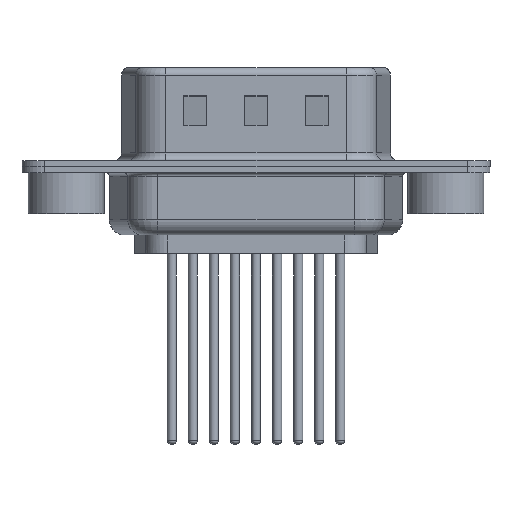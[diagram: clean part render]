
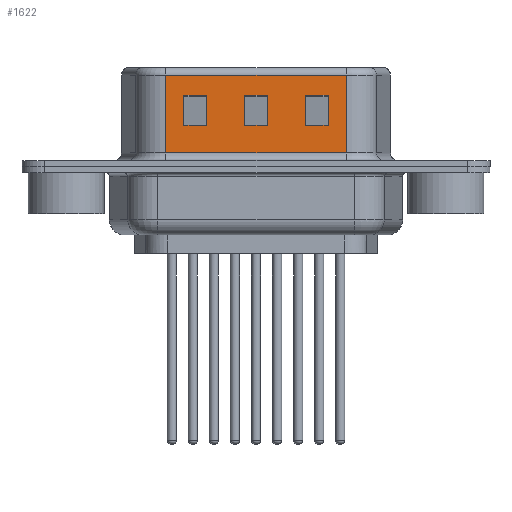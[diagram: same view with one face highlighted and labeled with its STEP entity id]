
A CAD part, front view. The second image highlights one B-rep face of the part: STEP entity #1622.
In plain terms, the highlighted planar face has unit normal (0, -1, 0).
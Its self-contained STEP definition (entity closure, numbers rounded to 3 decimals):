
#110 = CARTESIAN_POINT ( 'NONE',  ( 15.75, -4.55, 6.52 ) ) ;
#192 = CARTESIAN_POINT ( 'NONE',  ( 13.25, -4.55, 4.705 ) ) ;
#197 = EDGE_CURVE ( 'NONE', #6406, #1345, #12209, .T. ) ;
#223 = EDGE_CURVE ( 'NONE', #12306, #12247, #8976, .T. ) ;
#243 = CARTESIAN_POINT ( 'NONE',  ( 15.75, -4.55, 2.705 ) ) ;
#378 = DIRECTION ( 'NONE',  ( 1., 0., 0. ) ) ;
#596 = LINE ( 'NONE', #2812, #13760 ) ;
#843 = CARTESIAN_POINT ( 'NONE',  ( 13.25, -4.55, 6.52 ) ) ;
#916 = VERTEX_POINT ( 'NONE', #6265 ) ;
#1202 = FACE_OUTER_BOUND ( 'NONE', #9700, .T. ) ;
#1207 = EDGE_CURVE ( 'NONE', #12306, #9636, #13440, .T. ) ;
#1319 = LINE ( 'NONE', #5801, #10134 ) ;
#1322 = VECTOR ( 'NONE', #3563, 1000. ) ;
#1345 = VERTEX_POINT ( 'NONE', #10413 ) ;
#1435 = EDGE_CURVE ( 'NONE', #12232, #7040, #1764, .T. ) ;
#1436 = CARTESIAN_POINT ( 'NONE',  ( 7.75, -4.55, 6.52 ) ) ;
#1447 = VECTOR ( 'NONE', #6151, 1000. ) ;
#1486 = VECTOR ( 'NONE', #4485, 1000. ) ;
#1622 = ADVANCED_FACE ( 'NONE', ( #3118, #11858, #5326, #1202 ), #5608, .F. ) ;
#1712 = ORIENTED_EDGE ( 'NONE', *, *, #223, .T. ) ;
#1764 = LINE ( 'NONE', #9267, #13206 ) ;
#1804 = CARTESIAN_POINT ( 'NONE',  ( 14.451, -4.55, 2.705 ) ) ;
#1902 = ORIENTED_EDGE ( 'NONE', *, *, #7539, .T. ) ;
#1944 = VECTOR ( 'NONE', #9776, 1000. ) ;
#2072 = ORIENTED_EDGE ( 'NONE', *, *, #1435, .T. ) ;
#2132 = LINE ( 'NONE', #2281, #1486 ) ;
#2257 = CARTESIAN_POINT ( 'NONE',  ( 11.75, -4.55, 4.705 ) ) ;
#2281 = CARTESIAN_POINT ( 'NONE',  ( 14.451, -4.55, 4.705 ) ) ;
#2330 = LINE ( 'NONE', #13998, #5600 ) ;
#2370 = DIRECTION ( 'NONE',  ( -1., 0., 0. ) ) ;
#2619 = ORIENTED_EDGE ( 'NONE', *, *, #3644, .T. ) ;
#2812 = CARTESIAN_POINT ( 'NONE',  ( 18.451, -4.55, 2.705 ) ) ;
#2849 = LINE ( 'NONE', #843, #12120 ) ;
#2872 = LINE ( 'NONE', #1804, #1447 ) ;
#3118 = FACE_BOUND ( 'NONE', #3372, .T. ) ;
#3152 = VERTEX_POINT ( 'NONE', #192 ) ;
#3372 = EDGE_LOOP ( 'NONE', ( #10739, #12139, #14096, #11766 ) ) ;
#3445 = CARTESIAN_POINT ( 'NONE',  ( 22.451, -4.55, 2.705 ) ) ;
#3563 = DIRECTION ( 'NONE',  ( 0., 0., -1. ) ) ;
#3644 = EDGE_CURVE ( 'NONE', #3152, #11123, #2849, .T. ) ;
#3684 = CARTESIAN_POINT ( 'NONE',  ( 7.75, -4.55, 2.705 ) ) ;
#3952 = DIRECTION ( 'NONE',  ( -1., 0., 0. ) ) ;
#4174 = DIRECTION ( 'NONE',  ( 0., 0., -1. ) ) ;
#4263 = CARTESIAN_POINT ( 'NONE',  ( 17.25, -4.55, 2.705 ) ) ;
#4485 = DIRECTION ( 'NONE',  ( 1., 0., 0. ) ) ;
#4489 = VECTOR ( 'NONE', #11127, 1000. ) ;
#4613 = CARTESIAN_POINT ( 'NONE',  ( 18.451, -4.55, 6.02 ) ) ;
#4902 = VERTEX_POINT ( 'NONE', #9011 ) ;
#5326 = FACE_BOUND ( 'NONE', #9345, .T. ) ;
#5336 = CARTESIAN_POINT ( 'NONE',  ( 18.451, -4.55, 0.9 ) ) ;
#5466 = CARTESIAN_POINT ( 'NONE',  ( 13.25, -4.55, 2.705 ) ) ;
#5600 = VECTOR ( 'NONE', #4174, 1000. ) ;
#5608 = PLANE ( 'NONE',  #10463 ) ;
#5801 = CARTESIAN_POINT ( 'NONE',  ( 22.451, -4.55, 4.705 ) ) ;
#5897 = VERTEX_POINT ( 'NONE', #3684 ) ;
#5953 = VERTEX_POINT ( 'NONE', #12767 ) ;
#5986 = EDGE_CURVE ( 'NONE', #11123, #5953, #596, .T. ) ;
#6151 = DIRECTION ( 'NONE',  ( -1., 0., 0. ) ) ;
#6265 = CARTESIAN_POINT ( 'NONE',  ( 9.25, -4.55, 2.705 ) ) ;
#6348 = CARTESIAN_POINT ( 'NONE',  ( 9.25, -4.55, 6.52 ) ) ;
#6406 = VERTEX_POINT ( 'NONE', #243 ) ;
#6555 = ORIENTED_EDGE ( 'NONE', *, *, #5986, .T. ) ;
#6597 = EDGE_CURVE ( 'NONE', #916, #5897, #2872, .T. ) ;
#7040 = VERTEX_POINT ( 'NONE', #4263 ) ;
#7423 = CARTESIAN_POINT ( 'NONE',  ( 18.451, -4.55, 4.705 ) ) ;
#7434 = VERTEX_POINT ( 'NONE', #2257 ) ;
#7539 = EDGE_CURVE ( 'NONE', #1345, #12232, #1319, .T. ) ;
#7830 = DIRECTION ( 'NONE',  ( -1., 0., 0. ) ) ;
#7879 = ORIENTED_EDGE ( 'NONE', *, *, #1207, .F. ) ;
#8493 = DIRECTION ( 'NONE',  ( 1., 0., 0. ) ) ;
#8779 = VECTOR ( 'NONE', #2370, 1000. ) ;
#8802 = VECTOR ( 'NONE', #9848, 1000. ) ;
#8837 = VECTOR ( 'NONE', #7830, 1000. ) ;
#8976 = LINE ( 'NONE', #4613, #8837 ) ;
#9011 = CARTESIAN_POINT ( 'NONE',  ( 7.75, -4.55, 4.705 ) ) ;
#9044 = VERTEX_POINT ( 'NONE', #11496 ) ;
#9141 = EDGE_LOOP ( 'NONE', ( #2072, #10570, #11095, #1902 ) ) ;
#9267 = CARTESIAN_POINT ( 'NONE',  ( 17.25, -4.55, 6.52 ) ) ;
#9345 = EDGE_LOOP ( 'NONE', ( #14007, #2619, #6555, #12092 ) ) ;
#9632 = LINE ( 'NONE', #6348, #11775 ) ;
#9636 = VERTEX_POINT ( 'NONE', #11483 ) ;
#9700 = EDGE_LOOP ( 'NONE', ( #7879, #1712, #11494, #11023 ) ) ;
#9776 = DIRECTION ( 'NONE',  ( 0., 0., 1. ) ) ;
#9778 = VERTEX_POINT ( 'NONE', #10676 ) ;
#9848 = DIRECTION ( 'NONE',  ( 1., 0., 0. ) ) ;
#9939 = VECTOR ( 'NONE', #10222, 1000. ) ;
#10134 = VECTOR ( 'NONE', #378, 1000. ) ;
#10222 = DIRECTION ( 'NONE',  ( 0., 0., 1. ) ) ;
#10413 = CARTESIAN_POINT ( 'NONE',  ( 15.75, -4.55, 4.705 ) ) ;
#10463 = AXIS2_PLACEMENT_3D ( 'NONE', #12147, #13350, #11205 ) ;
#10570 = ORIENTED_EDGE ( 'NONE', *, *, #10783, .T. ) ;
#10676 = CARTESIAN_POINT ( 'NONE',  ( 9.25, -4.55, 4.705 ) ) ;
#10739 = ORIENTED_EDGE ( 'NONE', *, *, #11807, .T. ) ;
#10783 = EDGE_CURVE ( 'NONE', #7040, #6406, #11034, .T. ) ;
#10787 = LINE ( 'NONE', #5336, #8802 ) ;
#10860 = LINE ( 'NONE', #12088, #1944 ) ;
#11023 = ORIENTED_EDGE ( 'NONE', *, *, #12980, .T. ) ;
#11034 = LINE ( 'NONE', #3445, #8779 ) ;
#11095 = ORIENTED_EDGE ( 'NONE', *, *, #197, .T. ) ;
#11123 = VERTEX_POINT ( 'NONE', #5466 ) ;
#11127 = DIRECTION ( 'NONE',  ( 0., 0., 1. ) ) ;
#11205 = DIRECTION ( 'NONE',  ( 0., 0., 1. ) ) ;
#11483 = CARTESIAN_POINT ( 'NONE',  ( 18.451, -4.55, 0.9 ) ) ;
#11494 = ORIENTED_EDGE ( 'NONE', *, *, #13474, .T. ) ;
#11496 = CARTESIAN_POINT ( 'NONE',  ( 6.549, -4.55, 0.9 ) ) ;
#11527 = CARTESIAN_POINT ( 'NONE',  ( 6.549, -4.55, 6.02 ) ) ;
#11541 = VECTOR ( 'NONE', #8493, 1000. ) ;
#11747 = EDGE_CURVE ( 'NONE', #5897, #4902, #12530, .T. ) ;
#11766 = ORIENTED_EDGE ( 'NONE', *, *, #12942, .T. ) ;
#11775 = VECTOR ( 'NONE', #14026, 1000. ) ;
#11807 = EDGE_CURVE ( 'NONE', #9778, #916, #9632, .T. ) ;
#11827 = EDGE_CURVE ( 'NONE', #7434, #3152, #12744, .T. ) ;
#11858 = FACE_BOUND ( 'NONE', #9141, .T. ) ;
#12088 = CARTESIAN_POINT ( 'NONE',  ( 11.75, -4.55, 6.52 ) ) ;
#12092 = ORIENTED_EDGE ( 'NONE', *, *, #12936, .T. ) ;
#12120 = VECTOR ( 'NONE', #12519, 1000. ) ;
#12139 = ORIENTED_EDGE ( 'NONE', *, *, #6597, .T. ) ;
#12147 = CARTESIAN_POINT ( 'NONE',  ( 18.451, -4.55, 6.52 ) ) ;
#12209 = LINE ( 'NONE', #110, #4489 ) ;
#12232 = VERTEX_POINT ( 'NONE', #12606 ) ;
#12247 = VERTEX_POINT ( 'NONE', #11527 ) ;
#12306 = VERTEX_POINT ( 'NONE', #13893 ) ;
#12519 = DIRECTION ( 'NONE',  ( 0., 0., -1. ) ) ;
#12530 = LINE ( 'NONE', #1436, #9939 ) ;
#12606 = CARTESIAN_POINT ( 'NONE',  ( 17.25, -4.55, 4.705 ) ) ;
#12744 = LINE ( 'NONE', #7423, #11541 ) ;
#12767 = CARTESIAN_POINT ( 'NONE',  ( 11.75, -4.55, 2.705 ) ) ;
#12936 = EDGE_CURVE ( 'NONE', #5953, #7434, #10860, .T. ) ;
#12942 = EDGE_CURVE ( 'NONE', #4902, #9778, #2132, .T. ) ;
#12980 = EDGE_CURVE ( 'NONE', #9044, #9636, #10787, .T. ) ;
#13206 = VECTOR ( 'NONE', #13645, 1000. ) ;
#13350 = DIRECTION ( 'NONE',  ( 0., 1., 0. ) ) ;
#13365 = CARTESIAN_POINT ( 'NONE',  ( 18.451, -4.55, 6.52 ) ) ;
#13440 = LINE ( 'NONE', #13365, #1322 ) ;
#13474 = EDGE_CURVE ( 'NONE', #12247, #9044, #2330, .T. ) ;
#13645 = DIRECTION ( 'NONE',  ( 0., 0., -1. ) ) ;
#13760 = VECTOR ( 'NONE', #3952, 1000. ) ;
#13893 = CARTESIAN_POINT ( 'NONE',  ( 18.451, -4.55, 6.02 ) ) ;
#13998 = CARTESIAN_POINT ( 'NONE',  ( 6.549, -4.55, 6.52 ) ) ;
#14007 = ORIENTED_EDGE ( 'NONE', *, *, #11827, .T. ) ;
#14026 = DIRECTION ( 'NONE',  ( 0., 0., -1. ) ) ;
#14096 = ORIENTED_EDGE ( 'NONE', *, *, #11747, .T. ) ;
